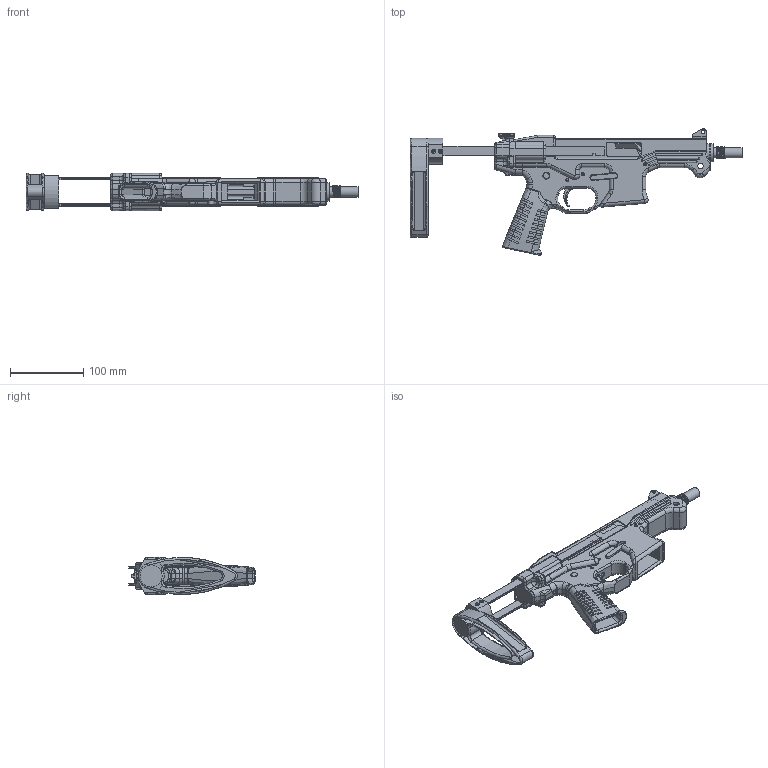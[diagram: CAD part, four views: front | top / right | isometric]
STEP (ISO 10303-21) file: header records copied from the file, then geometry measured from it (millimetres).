
FILE_DESCRIPTION(/* description */ (''),/* implementation_level */ '2;1');
FILE_NAME(/* name */ 'SVTR',/* author */ ('Logsleeve'),/* organization */ ('AWCY?'),/* authorisation */ '');
FILE_SCHEMA (('AUTOMOTIVE_DESIGN { 1 0 10303 214 3 1 1 }'));
Products named in the file (30): SVTR; SVTR_Receiver; VMAC9_Upper v2; SVTR_StockCover v3; SVTR_StockButton v2; Component2; SVTR_StockBar v2; SVTR_StockRail v4; SVTR_StockRail v4 (1); SVTR_TailhookAdapter v2; VMAC9_BCG v1; Ender_BedSpring v1; AR15_MagRelease v1; Magazine Catch Bar.step; Magazine Catch Button.step; Magazine Catch Spring.step; AR15_FCG v2; AR-15 Fire Control Group Full Auto.step; Fire Control Group.step; Hammer Assembly.step; Hammer Pin.step; Trigger Assembly.step; Trigger Disconnector.step; Trigger.step; Trigger Pin.step; Fire Selector Assembly.step; Fire Selector .step; Hammer.step; Tailhook v2; SVTR_FeedRamp v3
Assembly tree (30 placements, depth 6):
  SVTR
    SVTR_Receiver
    VMAC9_Upper v2
    SVTR_StockCover v3
    SVTR_StockButton v2
      Component2
    SVTR_StockBar v2
    SVTR_StockRail v4
    SVTR_StockRail v4 (1)
    SVTR_TailhookAdapter v2
    VMAC9_BCG v1
    Ender_BedSpring v1
    AR15_MagRelease v1
      Magazine Catch Bar.step
      Magazine Catch Button.step
      Magazine Catch Spring.step
    AR15_FCG v2
      AR-15 Fire Control Group Full Auto.step
        Fire Control Group.step
          Hammer Assembly.step
            Hammer.step
            Hammer Pin.step
          Trigger Assembly.step
            Trigger Disconnector.step
            Trigger.step
            Trigger Pin.step
          Fire Selector Assembly.step
            Fire Selector .step
      Hammer.step
    Tailhook v2
    SVTR_FeedRamp v3
Bounding box: 454.6 x 173.57 x 50.8 mm (x, y, z)
Volume: 600256.8 mm3; surface area: 258838.1 mm2
Topology: 23 solids, 23 shells, 2909 faces, 7829 edges, 4965 vertices
Faces by surface type: plane 1132, bspline 782, cylinder 677, torus 192, cone 65, sphere 61
Full cylindrical faces by diameter (mm): 2.5 x4, 2.7 x1, 2.946 x2, 3.023 x2, 3.4 x2, 3.5 x3, 3.556 x2, 3.858 x14, 3.912 x8, 3.962 x5, 4.039 x1, 4.064 x4, 4.216 x1, 4.318 x2, 4.4 x3, 4.5 x4, 4.572 x2, 4.712 x1, 4.727 x23, 5.08 x3, 5.182 x1, 5.715 x3, 5.842 x4, 6.35 x2, 7.62 x1, 7.874 x2, 7.95 x1, 7.986 x2, 8.128 x3, 8.255 x1
Entity records: 148230 total; most frequent: CARTESIAN_POINT 82597, ORIENTED_EDGE 14928, DIRECTION 11289, EDGE_CURVE 7464, VERTEX_POINT 4775, AXIS2_PLACEMENT_3D 3814, LINE 3661, VECTOR 3661
